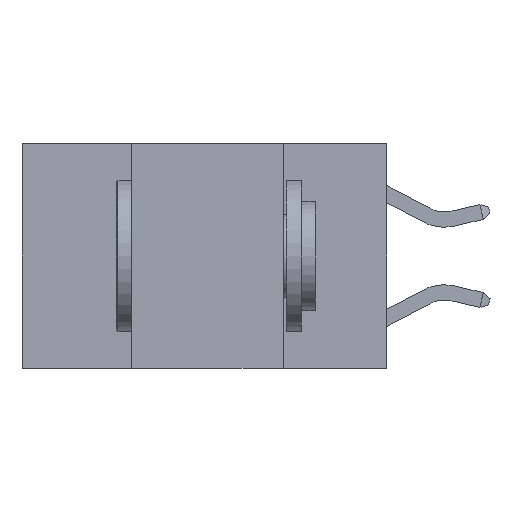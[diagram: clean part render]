
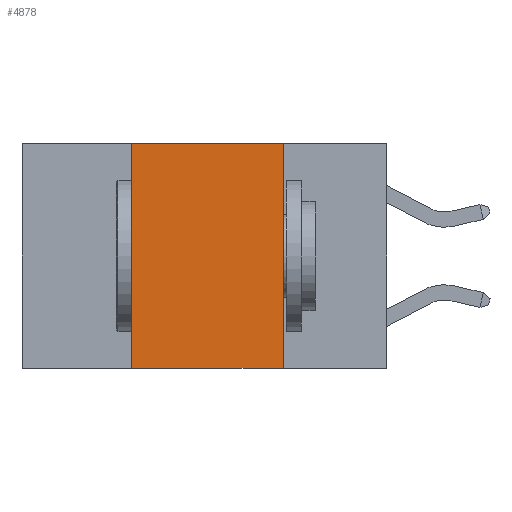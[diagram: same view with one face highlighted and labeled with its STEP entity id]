
A CAD part, left-side view. The second image highlights one B-rep face of the part: STEP entity #4878.
In plain terms, the highlighted planar face has unit normal (-1, 0, 0).
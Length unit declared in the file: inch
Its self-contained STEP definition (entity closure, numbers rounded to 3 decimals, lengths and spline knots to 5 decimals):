
#63 = CARTESIAN_POINT ( 'NONE',  ( 0., 0.6, -0.37 ) ) ;
#662 = VECTOR ( 'NONE', #28411, 39.37008 ) ;
#1102 = EDGE_CURVE ( 'NONE', #14191, #16395, #4331, .T. ) ;
#1258 = VECTOR ( 'NONE', #12190, 39.37008 ) ;
#2418 = ORIENTED_EDGE ( 'NONE', *, *, #18119, .F. ) ;
#2679 = EDGE_LOOP ( 'NONE', ( #18710, #17213, #2418, #18325 ) ) ;
#2913 = AXIS2_PLACEMENT_3D ( 'NONE', #3207, #19742, #5560 ) ;
#3207 = CARTESIAN_POINT ( 'NONE',  ( 0., 0.6, 0. ) ) ;
#3393 = CARTESIAN_POINT ( 'NONE',  ( 0., 0.42, -0.37 ) ) ;
#4331 = LINE ( 'NONE', #19251, #27952 ) ;
#4878 = ADVANCED_FACE ( 'NONE', ( #29041 ), #5450, .F. ) ;
#5450 = PLANE ( 'NONE',  #2913 ) ;
#5560 = DIRECTION ( 'NONE',  ( 0., 0., -1. ) ) ;
#6436 = EDGE_CURVE ( 'NONE', #16395, #10333, #12767, .T. ) ;
#7532 = LINE ( 'NONE', #21704, #1258 ) ;
#7621 = VERTEX_POINT ( 'NONE', #3393 ) ;
#10333 = VERTEX_POINT ( 'NONE', #10862 ) ;
#10862 = CARTESIAN_POINT ( 'NONE',  ( 0., 0.17, -0.37 ) ) ;
#10996 = DIRECTION ( 'NONE',  ( 0., 0., -1. ) ) ;
#12190 = DIRECTION ( 'NONE',  ( 0., 0., 1. ) ) ;
#12767 = LINE ( 'NONE', #15856, #23816 ) ;
#14191 = VERTEX_POINT ( 'NONE', #24466 ) ;
#15726 = CARTESIAN_POINT ( 'NONE',  ( 0., 0.17, 0. ) ) ;
#15856 = CARTESIAN_POINT ( 'NONE',  ( 0., 0.17, 0. ) ) ;
#16395 = VERTEX_POINT ( 'NONE', #15726 ) ;
#17213 = ORIENTED_EDGE ( 'NONE', *, *, #1102, .F. ) ;
#18119 = EDGE_CURVE ( 'NONE', #7621, #14191, #7532, .T. ) ;
#18325 = ORIENTED_EDGE ( 'NONE', *, *, #28720, .T. ) ;
#18710 = ORIENTED_EDGE ( 'NONE', *, *, #6436, .F. ) ;
#18861 = DIRECTION ( 'NONE',  ( 0., -1., 0. ) ) ;
#19251 = CARTESIAN_POINT ( 'NONE',  ( 0., 0.6, 0. ) ) ;
#19525 = LINE ( 'NONE', #63, #662 ) ;
#19742 = DIRECTION ( 'NONE',  ( 1., 0., 0. ) ) ;
#21704 = CARTESIAN_POINT ( 'NONE',  ( 0., 0.42, 0. ) ) ;
#23816 = VECTOR ( 'NONE', #10996, 39.37008 ) ;
#24466 = CARTESIAN_POINT ( 'NONE',  ( 0., 0.42, 0. ) ) ;
#27952 = VECTOR ( 'NONE', #18861, 39.37008 ) ;
#28411 = DIRECTION ( 'NONE',  ( 0., -1., 0. ) ) ;
#28720 = EDGE_CURVE ( 'NONE', #7621, #10333, #19525, .T. ) ;
#29041 = FACE_OUTER_BOUND ( 'NONE', #2679, .T. ) ;
